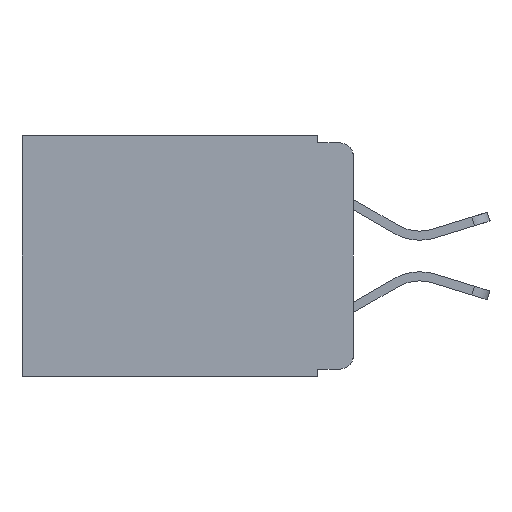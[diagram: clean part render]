
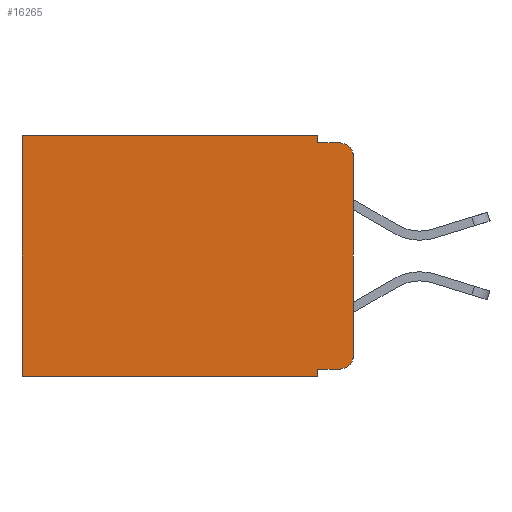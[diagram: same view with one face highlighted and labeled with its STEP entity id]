
A CAD part, left-side view. The second image highlights one B-rep face of the part: STEP entity #16265.
In plain terms, the highlighted planar face has unit normal (-1, 0, 0).
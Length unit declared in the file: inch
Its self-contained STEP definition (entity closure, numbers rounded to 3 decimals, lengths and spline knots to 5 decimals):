
#168 = DIRECTION ( 'NONE',  ( -1., 0., 0. ) ) ;
#362 = DIRECTION ( 'NONE',  ( 0., 1., 0. ) ) ;
#499 = CARTESIAN_POINT ( 'NONE',  ( 0.298, 0., -0.03 ) ) ;
#917 = VERTEX_POINT ( 'NONE', #19652 ) ;
#1131 = VERTEX_POINT ( 'NONE', #6096 ) ;
#1340 = EDGE_CURVE ( 'NONE', #917, #3227, #6488, .T. ) ;
#1604 = AXIS2_PLACEMENT_3D ( 'NONE', #2150, #168, #4958 ) ;
#1679 = DIRECTION ( 'NONE',  ( 0., 0., -1. ) ) ;
#1927 = LINE ( 'NONE', #23047, #16512 ) ;
#2052 = ORIENTED_EDGE ( 'NONE', *, *, #9425, .F. ) ;
#2150 = CARTESIAN_POINT ( 'NONE',  ( 0.298, 0.02, -0.313 ) ) ;
#2274 = LINE ( 'NONE', #18226, #6717 ) ;
#2797 = CIRCLE ( 'NONE', #12161, 0.02 ) ;
#3221 = ORIENTED_EDGE ( 'NONE', *, *, #18083, .T. ) ;
#3227 = VERTEX_POINT ( 'NONE', #13344 ) ;
#3311 = CARTESIAN_POINT ( 'NONE',  ( 0.298, 0.051, 0. ) ) ;
#3456 = ORIENTED_EDGE ( 'NONE', *, *, #1340, .T. ) ;
#3797 = CARTESIAN_POINT ( 'NONE',  ( 0.298, 0., 0. ) ) ;
#4809 = VECTOR ( 'NONE', #7712, 39.37008 ) ;
#4939 = ORIENTED_EDGE ( 'NONE', *, *, #14519, .T. ) ;
#4958 = DIRECTION ( 'NONE',  ( 0., 0., -1. ) ) ;
#5242 = DIRECTION ( 'NONE',  ( 0., 0., -1. ) ) ;
#5274 = VERTEX_POINT ( 'NONE', #15652 ) ;
#5988 = EDGE_CURVE ( 'NONE', #23940, #5274, #9255, .T. ) ;
#6096 = CARTESIAN_POINT ( 'NONE',  ( 0.298, 0.051, -0.333 ) ) ;
#6488 = CIRCLE ( 'NONE', #1604, 0.02 ) ;
#6717 = VECTOR ( 'NONE', #10694, 39.37008 ) ;
#7292 = ORIENTED_EDGE ( 'NONE', *, *, #13245, .T. ) ;
#7401 = VERTEX_POINT ( 'NONE', #499 ) ;
#7693 = VERTEX_POINT ( 'NONE', #14931 ) ;
#7712 = DIRECTION ( 'NONE',  ( 0., 1., 0. ) ) ;
#8057 = VECTOR ( 'NONE', #18339, 39.37008 ) ;
#8754 = DIRECTION ( 'NONE',  ( 0., -1., 0. ) ) ;
#8759 = LINE ( 'NONE', #23830, #22631 ) ;
#8899 = AXIS2_PLACEMENT_3D ( 'NONE', #3797, #22684, #11425 ) ;
#8922 = VECTOR ( 'NONE', #5242, 39.37008 ) ;
#9255 = LINE ( 'NONE', #18087, #23096 ) ;
#9425 = EDGE_CURVE ( 'NONE', #1131, #20886, #18732, .T. ) ;
#9434 = ORIENTED_EDGE ( 'NONE', *, *, #5988, .T. ) ;
#9492 = PLANE ( 'NONE',  #8899 ) ;
#9855 = CARTESIAN_POINT ( 'NONE',  ( 0.298, 0., 0. ) ) ;
#10086 = CARTESIAN_POINT ( 'NONE',  ( 0.298, 0.051, -0.343 ) ) ;
#10281 = CARTESIAN_POINT ( 'NONE',  ( 0.298, 0.473, 0. ) ) ;
#10694 = DIRECTION ( 'NONE',  ( 0., -1., 0. ) ) ;
#11425 = DIRECTION ( 'NONE',  ( 0., 0., -1. ) ) ;
#11568 = CARTESIAN_POINT ( 'NONE',  ( 0.298, 0.051, 0. ) ) ;
#12161 = AXIS2_PLACEMENT_3D ( 'NONE', #24290, #13063, #1679 ) ;
#12353 = ORIENTED_EDGE ( 'NONE', *, *, #20157, .F. ) ;
#12644 = EDGE_CURVE ( 'NONE', #7693, #20503, #2274, .T. ) ;
#12684 = DIRECTION ( 'NONE',  ( 0., 0., -1. ) ) ;
#12744 = EDGE_LOOP ( 'NONE', ( #16324, #4939, #20309, #22698, #3221, #9434, #12353, #2052, #7292, #3456 ) ) ;
#13063 = DIRECTION ( 'NONE',  ( -1., 0., 0. ) ) ;
#13245 = EDGE_CURVE ( 'NONE', #1131, #917, #8759, .T. ) ;
#13344 = CARTESIAN_POINT ( 'NONE',  ( 0.298, 0., -0.313 ) ) ;
#13368 = FACE_OUTER_BOUND ( 'NONE', #12744, .T. ) ;
#13592 = DIRECTION ( 'NONE',  ( 0., 0., -1. ) ) ;
#14519 = EDGE_CURVE ( 'NONE', #7401, #20503, #2797, .T. ) ;
#14905 = LINE ( 'NONE', #19057, #4809 ) ;
#14931 = CARTESIAN_POINT ( 'NONE',  ( 0.298, 0.051, -0.01 ) ) ;
#15286 = LINE ( 'NONE', #9855, #20290 ) ;
#15652 = CARTESIAN_POINT ( 'NONE',  ( 0.298, 0.473, -0.343 ) ) ;
#16265 = ADVANCED_FACE ( 'NONE', ( #13368 ), #9492, .F. ) ;
#16324 = ORIENTED_EDGE ( 'NONE', *, *, #16909, .F. ) ;
#16512 = VECTOR ( 'NONE', #362, 39.37008 ) ;
#16909 = EDGE_CURVE ( 'NONE', #7401, #3227, #15286, .T. ) ;
#18083 = EDGE_CURVE ( 'NONE', #24079, #23940, #14905, .T. ) ;
#18087 = CARTESIAN_POINT ( 'NONE',  ( 0.298, 0.473, 0. ) ) ;
#18161 = CARTESIAN_POINT ( 'NONE',  ( 0.298, 0.051, 0. ) ) ;
#18226 = CARTESIAN_POINT ( 'NONE',  ( 0.298, 0.051, -0.01 ) ) ;
#18339 = DIRECTION ( 'NONE',  ( 0., 0., -1. ) ) ;
#18732 = LINE ( 'NONE', #11568, #8057 ) ;
#19057 = CARTESIAN_POINT ( 'NONE',  ( 0.298, 0., 0. ) ) ;
#19567 = LINE ( 'NONE', #3311, #8922 ) ;
#19652 = CARTESIAN_POINT ( 'NONE',  ( 0.298, 0.02, -0.333 ) ) ;
#20157 = EDGE_CURVE ( 'NONE', #20886, #5274, #1927, .T. ) ;
#20290 = VECTOR ( 'NONE', #13592, 39.37008 ) ;
#20309 = ORIENTED_EDGE ( 'NONE', *, *, #12644, .F. ) ;
#20503 = VERTEX_POINT ( 'NONE', #22232 ) ;
#20886 = VERTEX_POINT ( 'NONE', #10086 ) ;
#22232 = CARTESIAN_POINT ( 'NONE',  ( 0.298, 0.02, -0.01 ) ) ;
#22450 = EDGE_CURVE ( 'NONE', #24079, #7693, #19567, .T. ) ;
#22631 = VECTOR ( 'NONE', #8754, 39.37008 ) ;
#22684 = DIRECTION ( 'NONE',  ( 1., 0., 0. ) ) ;
#22698 = ORIENTED_EDGE ( 'NONE', *, *, #22450, .F. ) ;
#23047 = CARTESIAN_POINT ( 'NONE',  ( 0.298, 0., -0.343 ) ) ;
#23096 = VECTOR ( 'NONE', #12684, 39.37008 ) ;
#23830 = CARTESIAN_POINT ( 'NONE',  ( 0.298, 0.051, -0.333 ) ) ;
#23940 = VERTEX_POINT ( 'NONE', #10281 ) ;
#24079 = VERTEX_POINT ( 'NONE', #18161 ) ;
#24290 = CARTESIAN_POINT ( 'NONE',  ( 0.298, 0.02, -0.03 ) ) ;
